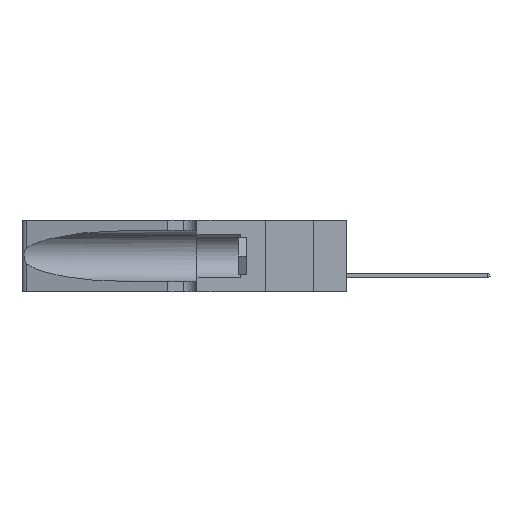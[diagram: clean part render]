
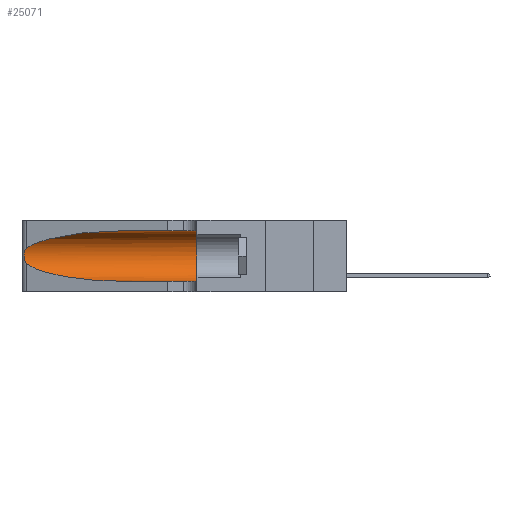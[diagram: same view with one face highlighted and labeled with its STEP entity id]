
A CAD part, left-side view. The second image highlights one B-rep face of the part: STEP entity #25071.
In plain terms, the highlighted cylindrical face has radius 3.308 mm (diameter 6.617 mm), a partial arc.
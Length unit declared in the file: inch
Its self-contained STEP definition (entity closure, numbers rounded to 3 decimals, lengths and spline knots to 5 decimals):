
#1417 = CARTESIAN_POINT ( 'NONE',  ( 0.18966, 0.96281, 0.31525 ) ) ;
#2711 = FACE_OUTER_BOUND ( 'NONE', #21733, .T. ) ;
#3826 = CARTESIAN_POINT ( 'NONE',  ( 0.26017, 1.23833, 0.17102 ) ) ;
#5101 = CARTESIAN_POINT ( 'NONE',  ( 0.25487, 1.22718, 0.22369 ) ) ;
#5217 = CARTESIAN_POINT ( 'NONE',  ( 0.25487, 1.22718, 0.14631 ) ) ;
#6444 = CARTESIAN_POINT ( 'NONE',  ( 0.1305, 0.72297, 0.31525 ) ) ;
#7158 = LINE ( 'NONE', #23627, #34266 ) ;
#8041 = DIRECTION ( 'NONE',  ( 0., -1., 0. ) ) ;
#8853 = CARTESIAN_POINT ( 'NONE',  ( 0.25789, 1.23486, 0.15765 ) ) ;
#9341 = CARTESIAN_POINT ( 'NONE',  ( 0.25555, 1.22994, 0.2215 ) ) ;
#9643 = VERTEX_POINT ( 'NONE', #16955 ) ;
#10285 = B_SPLINE_CURVE_WITH_KNOTS ( 'NONE', 3,
 ( #30461, #9341, #27412, #11733, #33302, #17323, #19769, #33194, #3826, #30350, #8853, #17210, #27526, #32821 ),
 .UNSPECIFIED., .F., .F.,
 ( 4, 2, 2, 2, 2, 2, 4 ),
 ( 0., 0.00027, 0.00053, 0.00107, 0.0016, 0.00187, 0.00214 ),
 .UNSPECIFIED. ) ;
#10583 = CARTESIAN_POINT ( 'NONE',  ( 0.1305, 0.72297, 0.05475 ) ) ;
#10972 = VECTOR ( 'NONE', #18695, 39.37008 ) ;
#11510 = DIRECTION ( 'NONE',  ( 0., 0., -1. ) ) ;
#11733 = CARTESIAN_POINT ( 'NONE',  ( 0.25787, 1.23484, 0.2124 ) ) ;
#11908 = CYLINDRICAL_SURFACE ( 'NONE', #27420, 0.13025 ) ;
#12148 = ORIENTED_EDGE ( 'NONE', *, *, #29512, .F. ) ;
#12464 = DIRECTION ( 'NONE',  ( 0., 1., 0. ) ) ;
#12668 = ORIENTED_EDGE ( 'NONE', *, *, #18015, .T. ) ;
#12842 = CARTESIAN_POINT ( 'NONE',  ( 0.1305, 0.35, 0.05475 ) ) ;
#13124 = CARTESIAN_POINT ( 'NONE',  ( 0.2373, 1.15595, 0.08982 ) ) ;
#13275 = CARTESIAN_POINT ( 'NONE',  ( 0.25487, 1.22718, 0.22369 ) ) ;
#13345 = ORIENTED_EDGE ( 'NONE', *, *, #16875, .F. ) ;
#13833 =( BOUNDED_CURVE ( )  B_SPLINE_CURVE ( 3, ( #5217, #13124, #31760, #10583 ),
 .UNSPECIFIED., .F., .F. ) 
 B_SPLINE_CURVE_WITH_KNOTS ( ( 4, 4 ),
 ( 3.44316, 4.71239 ),
 .UNSPECIFIED. ) 
 CURVE ( )  GEOMETRIC_REPRESENTATION_ITEM ( )  RATIONAL_B_SPLINE_CURVE ( ( 1., 0.87, 0.87, 1. ) ) 
 REPRESENTATION_ITEM ( '' )  );
#15194 = VERTEX_POINT ( 'NONE', #5101 ) ;
#15370 = DIRECTION ( 'NONE',  ( 0., 0., 1. ) ) ;
#15374 = EDGE_CURVE ( 'NONE', #15194, #9643, #10285, .T. ) ;
#15583 = LINE ( 'NONE', #16135, #10972 ) ;
#16135 = CARTESIAN_POINT ( 'NONE',  ( 0.1305, 1.61858, 0.05475 ) ) ;
#16856 =( BOUNDED_CURVE ( )  B_SPLINE_CURVE ( 3, ( #6444, #1417, #18951, #13275 ),
 .UNSPECIFIED., .F., .T. ) 
 B_SPLINE_CURVE_WITH_KNOTS ( ( 4, 4 ),
 ( 1.5708, 2.84003 ),
 .UNSPECIFIED. ) 
 CURVE ( )  GEOMETRIC_REPRESENTATION_ITEM ( )  RATIONAL_B_SPLINE_CURVE ( ( 1., 0.87, 0.87, 1. ) ) 
 REPRESENTATION_ITEM ( '' )  );
#16875 = EDGE_CURVE ( 'NONE', #17647, #23666, #7158, .T. ) ;
#16955 = CARTESIAN_POINT ( 'NONE',  ( 0.25487, 1.22718, 0.14631 ) ) ;
#17210 = CARTESIAN_POINT ( 'NONE',  ( 0.25639, 1.23186, 0.15144 ) ) ;
#17323 = CARTESIAN_POINT ( 'NONE',  ( 0.26018, 1.23835, 0.19895 ) ) ;
#17647 = VERTEX_POINT ( 'NONE', #24991 ) ;
#18015 = EDGE_CURVE ( 'NONE', #17647, #15194, #16856, .T. ) ;
#18235 = CIRCLE ( 'NONE', #21276, 0.13025 ) ;
#18253 = ORIENTED_EDGE ( 'NONE', *, *, #25916, .T. ) ;
#18695 = DIRECTION ( 'NONE',  ( 0., -1., 0. ) ) ;
#18951 = CARTESIAN_POINT ( 'NONE',  ( 0.2373, 1.15595, 0.28018 ) ) ;
#19537 = DIRECTION ( 'NONE',  ( 0., -1., 0. ) ) ;
#19769 = CARTESIAN_POINT ( 'NONE',  ( 0.26075, 1.23896, 0.19203 ) ) ;
#20866 = VERTEX_POINT ( 'NONE', #31807 ) ;
#21276 = AXIS2_PLACEMENT_3D ( 'NONE', #31322, #12464, #15370 ) ;
#21733 = EDGE_LOOP ( 'NONE', ( #12668, #29548, #32257, #18253, #12148, #13345 ) ) ;
#21847 = CARTESIAN_POINT ( 'NONE',  ( 0.1305, 1.61858, 0.185 ) ) ;
#23627 = CARTESIAN_POINT ( 'NONE',  ( 0.1305, 1.61858, 0.31525 ) ) ;
#23666 = VERTEX_POINT ( 'NONE', #31261 ) ;
#24991 = CARTESIAN_POINT ( 'NONE',  ( 0.1305, 0.72297, 0.31525 ) ) ;
#25071 = ADVANCED_FACE ( 'NONE', ( #2711 ), #11908, .F. ) ;
#25916 = EDGE_CURVE ( 'NONE', #20866, #28517, #15583, .T. ) ;
#27412 = CARTESIAN_POINT ( 'NONE',  ( 0.25639, 1.23184, 0.21858 ) ) ;
#27420 = AXIS2_PLACEMENT_3D ( 'NONE', #21847, #19537, #11510 ) ;
#27526 = CARTESIAN_POINT ( 'NONE',  ( 0.25555, 1.22993, 0.14849 ) ) ;
#28517 = VERTEX_POINT ( 'NONE', #12842 ) ;
#29512 = EDGE_CURVE ( 'NONE', #23666, #28517, #18235, .T. ) ;
#29548 = ORIENTED_EDGE ( 'NONE', *, *, #15374, .T. ) ;
#29657 = EDGE_CURVE ( 'NONE', #9643, #20866, #13833, .T. ) ;
#30350 = CARTESIAN_POINT ( 'NONE',  ( 0.25856, 1.23593, 0.16098 ) ) ;
#30461 = CARTESIAN_POINT ( 'NONE',  ( 0.25487, 1.22718, 0.22369 ) ) ;
#31261 = CARTESIAN_POINT ( 'NONE',  ( 0.1305, 0.35, 0.31525 ) ) ;
#31322 = CARTESIAN_POINT ( 'NONE',  ( 0.1305, 0.35, 0.185 ) ) ;
#31760 = CARTESIAN_POINT ( 'NONE',  ( 0.18966, 0.96281, 0.05475 ) ) ;
#31807 = CARTESIAN_POINT ( 'NONE',  ( 0.1305, 0.72297, 0.05475 ) ) ;
#32257 = ORIENTED_EDGE ( 'NONE', *, *, #29657, .T. ) ;
#32821 = CARTESIAN_POINT ( 'NONE',  ( 0.25487, 1.22718, 0.14631 ) ) ;
#33194 = CARTESIAN_POINT ( 'NONE',  ( 0.26075, 1.23896, 0.178 ) ) ;
#33302 = CARTESIAN_POINT ( 'NONE',  ( 0.25854, 1.2359, 0.20912 ) ) ;
#34266 = VECTOR ( 'NONE', #8041, 39.37008 ) ;
